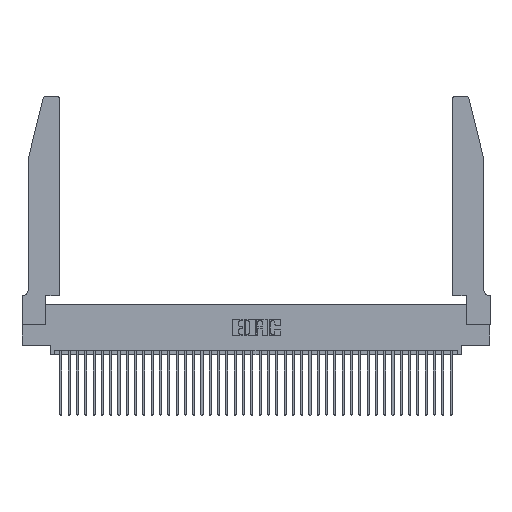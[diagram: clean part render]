
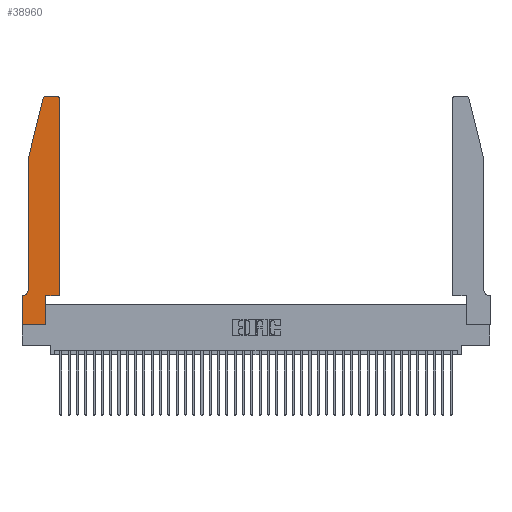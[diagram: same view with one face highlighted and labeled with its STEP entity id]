
A CAD part, top view. The second image highlights one B-rep face of the part: STEP entity #38960.
In plain terms, the highlighted planar face has unit normal (0, 0, 1).
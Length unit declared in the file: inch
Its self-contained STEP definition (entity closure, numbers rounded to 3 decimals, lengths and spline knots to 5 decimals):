
#575 = VECTOR ( 'NONE', #23158, 39.37008 ) ;
#587 = LINE ( 'NONE', #3755, #25341 ) ;
#805 = ORIENTED_EDGE ( 'NONE', *, *, #25181, .T. ) ;
#843 = VERTEX_POINT ( 'NONE', #7844 ) ;
#967 = VECTOR ( 'NONE', #21634, 39.37008 ) ;
#1031 = DIRECTION ( 'NONE',  ( 0., 0., 1. ) ) ;
#1063 = EDGE_CURVE ( 'NONE', #843, #6965, #11662, .T. ) ;
#1289 = VERTEX_POINT ( 'NONE', #41211 ) ;
#1365 = ORIENTED_EDGE ( 'NONE', *, *, #23975, .T. ) ;
#2581 = ORIENTED_EDGE ( 'NONE', *, *, #4611, .T. ) ;
#2765 = CARTESIAN_POINT ( 'NONE',  ( 0.284, 2.72, 0.37 ) ) ;
#2782 = CARTESIAN_POINT ( 'NONE',  ( 0.4505, 0.35, 0.37 ) ) ;
#3300 = CARTESIAN_POINT ( 'NONE',  ( 0.0755, 2., 0.37 ) ) ;
#3444 = ORIENTED_EDGE ( 'NONE', *, *, #36555, .T. ) ;
#3457 = LINE ( 'NONE', #25062, #7474 ) ;
#3755 = CARTESIAN_POINT ( 'NONE',  ( 0.2865, 0.35, 0.37 ) ) ;
#3779 = VECTOR ( 'NONE', #39656, 39.37008 ) ;
#3782 = CARTESIAN_POINT ( 'NONE',  ( 0.2865, 0.35, 0.37 ) ) ;
#4611 = EDGE_CURVE ( 'NONE', #19551, #1289, #5806, .T. ) ;
#4770 = CARTESIAN_POINT ( 'NONE',  ( 0.4505, 0.35, 0.37 ) ) ;
#5381 = VERTEX_POINT ( 'NONE', #2782 ) ;
#5440 = EDGE_CURVE ( 'NONE', #23522, #21037, #22393, .T. ) ;
#5454 = AXIS2_PLACEMENT_3D ( 'NONE', #24174, #36735, #23880 ) ;
#5806 = CIRCLE ( 'NONE', #37590, 0.03 ) ;
#6306 = VERTEX_POINT ( 'NONE', #18833 ) ;
#6643 = EDGE_CURVE ( 'NONE', #20371, #5381, #22753, .T. ) ;
#6965 = VERTEX_POINT ( 'NONE', #23244 ) ;
#7474 = VECTOR ( 'NONE', #18176, 39.37008 ) ;
#7844 = CARTESIAN_POINT ( 'NONE',  ( 0.284, 2.75, 0.37 ) ) ;
#8070 = LINE ( 'NONE', #9461, #39895 ) ;
#8275 = CARTESIAN_POINT ( 'NONE',  ( 0., 0., 0.37 ) ) ;
#8810 = EDGE_CURVE ( 'NONE', #6306, #30701, #3457, .T. ) ;
#9222 = VECTOR ( 'NONE', #40408, 39.37008 ) ;
#9461 = CARTESIAN_POINT ( 'NONE',  ( 0.0755, 2., 0.37 ) ) ;
#11413 = ORIENTED_EDGE ( 'NONE', *, *, #17257, .T. ) ;
#11662 = CIRCLE ( 'NONE', #12154, 0.03 ) ;
#11876 = DIRECTION ( 'NONE',  ( 0., 0., 1. ) ) ;
#12154 = AXIS2_PLACEMENT_3D ( 'NONE', #2765, #38184, #18695 ) ;
#12285 = LINE ( 'NONE', #8275, #35486 ) ;
#12711 = VECTOR ( 'NONE', #25541, 39.37008 ) ;
#13363 = AXIS2_PLACEMENT_3D ( 'NONE', #24025, #1031, #30572 ) ;
#14124 = LINE ( 'NONE', #4770, #967 ) ;
#15263 = CARTESIAN_POINT ( 'NONE',  ( 0.4205, 2.72, 0.37 ) ) ;
#15550 = ORIENTED_EDGE ( 'NONE', *, *, #8810, .T. ) ;
#16537 = ORIENTED_EDGE ( 'NONE', *, *, #36963, .T. ) ;
#17076 = FACE_OUTER_BOUND ( 'NONE', #36074, .T. ) ;
#17257 = EDGE_CURVE ( 'NONE', #21037, #6306, #23807, .T. ) ;
#17797 = CARTESIAN_POINT ( 'NONE',  ( 0.2605, 2.75, 0.37 ) ) ;
#18006 = DIRECTION ( 'NONE',  ( 1., 0., 0. ) ) ;
#18176 = DIRECTION ( 'NONE',  ( 0., -1., 0. ) ) ;
#18447 = ORIENTED_EDGE ( 'NONE', *, *, #5440, .T. ) ;
#18695 = DIRECTION ( 'NONE',  ( 1., 0., 0. ) ) ;
#18791 = LINE ( 'NONE', #17797, #9222 ) ;
#18833 = CARTESIAN_POINT ( 'NONE',  ( 0., 0.35, 0.37 ) ) ;
#19551 = VERTEX_POINT ( 'NONE', #39813 ) ;
#19770 = CARTESIAN_POINT ( 'NONE',  ( 0.0755, 0.35, 0.37 ) ) ;
#19780 = ORIENTED_EDGE ( 'NONE', *, *, #1063, .T. ) ;
#20371 = VERTEX_POINT ( 'NONE', #3782 ) ;
#21037 = VERTEX_POINT ( 'NONE', #28739 ) ;
#21634 = DIRECTION ( 'NONE',  ( 0., 1., 0. ) ) ;
#22215 = CARTESIAN_POINT ( 'NONE',  ( 0.2865, 0., 0.37 ) ) ;
#22393 = CIRCLE ( 'NONE', #5454, 0.07 ) ;
#22753 = LINE ( 'NONE', #35762, #12711 ) ;
#22833 = ORIENTED_EDGE ( 'NONE', *, *, #6643, .T. ) ;
#23158 = DIRECTION ( 'NONE',  ( -1., 0., 0. ) ) ;
#23244 = CARTESIAN_POINT ( 'NONE',  ( 0.25487, 2.72718, 0.37 ) ) ;
#23522 = VERTEX_POINT ( 'NONE', #37326 ) ;
#23807 = LINE ( 'NONE', #19770, #575 ) ;
#23880 = DIRECTION ( 'NONE',  ( -1., 0., 0. ) ) ;
#23975 = EDGE_CURVE ( 'NONE', #1289, #843, #18791, .T. ) ;
#24025 = CARTESIAN_POINT ( 'NONE',  ( 0., 0.35, 0.37 ) ) ;
#24174 = CARTESIAN_POINT ( 'NONE',  ( 0.0055, 0.42, 0.37 ) ) ;
#25062 = CARTESIAN_POINT ( 'NONE',  ( 0., 0., 0.37 ) ) ;
#25181 = EDGE_CURVE ( 'NONE', #6965, #37629, #8070, .T. ) ;
#25341 = VECTOR ( 'NONE', #29991, 39.37008 ) ;
#25382 = EDGE_CURVE ( 'NONE', #5381, #19551, #14124, .T. ) ;
#25541 = DIRECTION ( 'NONE',  ( 1., 0., 0. ) ) ;
#27795 = DIRECTION ( 'NONE',  ( 1., 0., 0. ) ) ;
#28739 = CARTESIAN_POINT ( 'NONE',  ( 0.0055, 0.35, 0.37 ) ) ;
#29991 = DIRECTION ( 'NONE',  ( 0., 1., 0. ) ) ;
#30572 = DIRECTION ( 'NONE',  ( 1., 0., 0. ) ) ;
#30701 = VERTEX_POINT ( 'NONE', #31658 ) ;
#31051 = ORIENTED_EDGE ( 'NONE', *, *, #32373, .T. ) ;
#31658 = CARTESIAN_POINT ( 'NONE',  ( 0., 0., 0.37 ) ) ;
#32373 = EDGE_CURVE ( 'NONE', #37629, #23522, #33588, .T. ) ;
#33588 = LINE ( 'NONE', #36412, #3779 ) ;
#34277 = DIRECTION ( 'NONE',  ( -0.239, -0.971, 0. ) ) ;
#35486 = VECTOR ( 'NONE', #18006, 39.37008 ) ;
#35762 = CARTESIAN_POINT ( 'NONE',  ( 0.4505, 0.35, 0.37 ) ) ;
#36074 = EDGE_LOOP ( 'NONE', ( #1365, #19780, #805, #31051, #18447, #11413, #15550, #3444, #16537, #22833, #38612, #2581 ) ) ;
#36412 = CARTESIAN_POINT ( 'NONE',  ( 0.0755, 2., 0.37 ) ) ;
#36555 = EDGE_CURVE ( 'NONE', #30701, #39901, #12285, .T. ) ;
#36735 = DIRECTION ( 'NONE',  ( 0., 0., -1. ) ) ;
#36891 = PLANE ( 'NONE',  #13363 ) ;
#36963 = EDGE_CURVE ( 'NONE', #39901, #20371, #587, .T. ) ;
#37326 = CARTESIAN_POINT ( 'NONE',  ( 0.0755, 0.42, 0.37 ) ) ;
#37590 = AXIS2_PLACEMENT_3D ( 'NONE', #15263, #11876, #27795 ) ;
#37629 = VERTEX_POINT ( 'NONE', #3300 ) ;
#38184 = DIRECTION ( 'NONE',  ( 0., 0., 1. ) ) ;
#38612 = ORIENTED_EDGE ( 'NONE', *, *, #25382, .T. ) ;
#38960 = ADVANCED_FACE ( 'NONE', ( #17076 ), #36891, .T. ) ;
#39656 = DIRECTION ( 'NONE',  ( 0., -1., 0. ) ) ;
#39813 = CARTESIAN_POINT ( 'NONE',  ( 0.4505, 2.72, 0.37 ) ) ;
#39895 = VECTOR ( 'NONE', #34277, 39.37008 ) ;
#39901 = VERTEX_POINT ( 'NONE', #22215 ) ;
#40408 = DIRECTION ( 'NONE',  ( -1., 0., 0. ) ) ;
#41211 = CARTESIAN_POINT ( 'NONE',  ( 0.4205, 2.75, 0.37 ) ) ;
